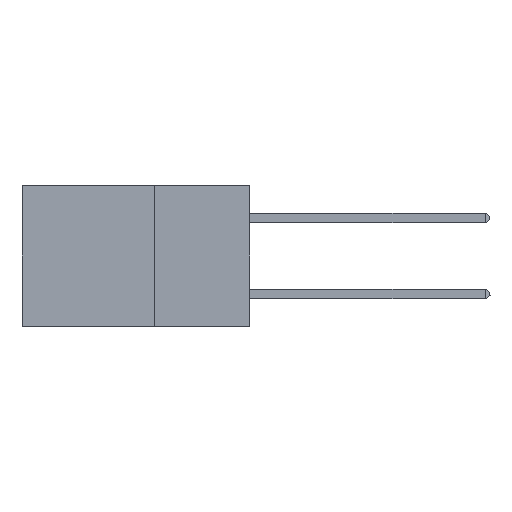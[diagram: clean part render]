
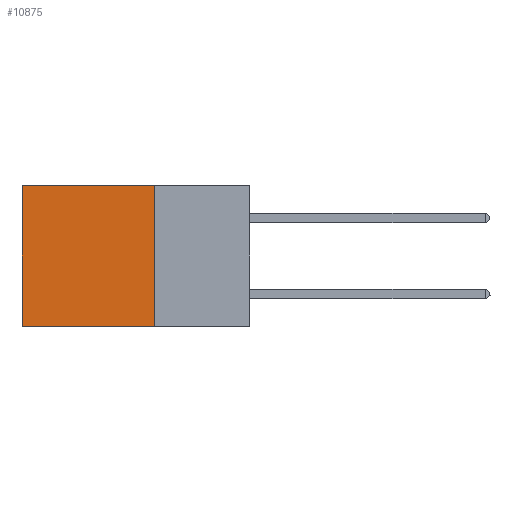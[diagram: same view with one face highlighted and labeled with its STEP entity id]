
A CAD part, left-side view. The second image highlights one B-rep face of the part: STEP entity #10875.
In plain terms, the highlighted planar face has unit normal (-1, 0, 0).
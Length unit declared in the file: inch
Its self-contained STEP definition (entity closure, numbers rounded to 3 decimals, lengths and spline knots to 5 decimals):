
#644 = EDGE_LOOP ( 'NONE', ( #2325, #34021, #2415, #21916 ) ) ;
#2098 = VERTEX_POINT ( 'NONE', #31228 ) ;
#2325 = ORIENTED_EDGE ( 'NONE', *, *, #4343, .T. ) ;
#2415 = ORIENTED_EDGE ( 'NONE', *, *, #4885, .F. ) ;
#4343 = EDGE_CURVE ( 'NONE', #10743, #2098, #24415, .T. ) ;
#4885 = EDGE_CURVE ( 'NONE', #24400, #14516, #16280, .T. ) ;
#5395 = DIRECTION ( 'NONE',  ( 0., 1., 0. ) ) ;
#8799 = CARTESIAN_POINT ( 'NONE',  ( 0.2875, 0.25, 0. ) ) ;
#10631 = DIRECTION ( 'NONE',  ( 0., 0., -1. ) ) ;
#10743 = VERTEX_POINT ( 'NONE', #19272 ) ;
#10875 = ADVANCED_FACE ( 'NONE', ( #12818 ), #34855, .F. ) ;
#11528 = CARTESIAN_POINT ( 'NONE',  ( 0.2875, 0.25, 0. ) ) ;
#12818 = FACE_OUTER_BOUND ( 'NONE', #644, .T. ) ;
#13762 = VECTOR ( 'NONE', #19667, 39.37008 ) ;
#14516 = VERTEX_POINT ( 'NONE', #32381 ) ;
#15490 = VECTOR ( 'NONE', #10631, 39.37008 ) ;
#15617 = LINE ( 'NONE', #8799, #24949 ) ;
#16133 = CARTESIAN_POINT ( 'NONE',  ( 0.2875, 0.25, -0.37 ) ) ;
#16280 = LINE ( 'NONE', #22520, #13762 ) ;
#16913 = EDGE_CURVE ( 'NONE', #14516, #2098, #33664, .T. ) ;
#18079 = VECTOR ( 'NONE', #5395, 39.37008 ) ;
#18423 = CARTESIAN_POINT ( 'NONE',  ( 0.2875, 0.6, 0. ) ) ;
#18741 = CARTESIAN_POINT ( 'NONE',  ( 0.2875, 0.25, 0. ) ) ;
#19272 = CARTESIAN_POINT ( 'NONE',  ( 0.2875, 0.6, 0. ) ) ;
#19667 = DIRECTION ( 'NONE',  ( 0., 0., -1. ) ) ;
#21584 = DIRECTION ( 'NONE',  ( 0., 0., -1. ) ) ;
#21916 = ORIENTED_EDGE ( 'NONE', *, *, #31942, .T. ) ;
#22520 = CARTESIAN_POINT ( 'NONE',  ( 0.2875, 0.25, 0. ) ) ;
#24400 = VERTEX_POINT ( 'NONE', #11528 ) ;
#24415 = LINE ( 'NONE', #18423, #15490 ) ;
#24653 = AXIS2_PLACEMENT_3D ( 'NONE', #18741, #26880, #21584 ) ;
#24949 = VECTOR ( 'NONE', #27678, 39.37008 ) ;
#26880 = DIRECTION ( 'NONE',  ( 1., 0., 0. ) ) ;
#27678 = DIRECTION ( 'NONE',  ( 0., 1., 0. ) ) ;
#31228 = CARTESIAN_POINT ( 'NONE',  ( 0.2875, 0.6, -0.37 ) ) ;
#31942 = EDGE_CURVE ( 'NONE', #24400, #10743, #15617, .T. ) ;
#32381 = CARTESIAN_POINT ( 'NONE',  ( 0.2875, 0.25, -0.37 ) ) ;
#33664 = LINE ( 'NONE', #16133, #18079 ) ;
#34021 = ORIENTED_EDGE ( 'NONE', *, *, #16913, .F. ) ;
#34855 = PLANE ( 'NONE',  #24653 ) ;
